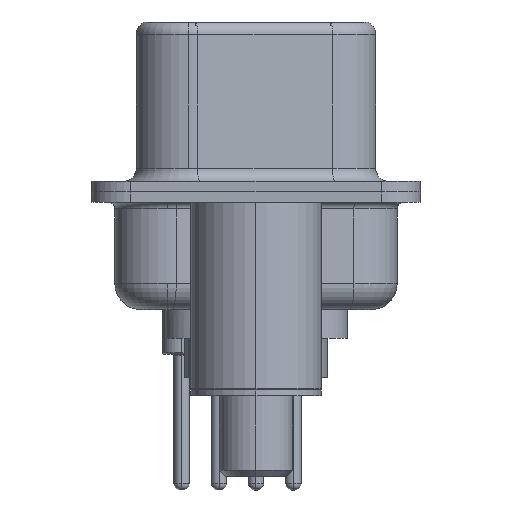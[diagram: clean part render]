
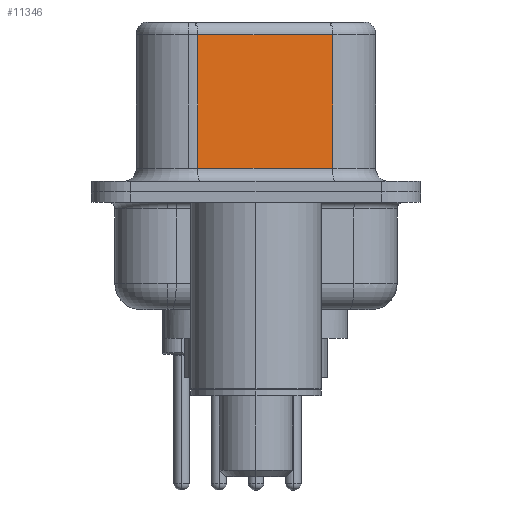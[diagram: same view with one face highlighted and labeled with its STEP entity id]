
A CAD part, left-side view. The second image highlights one B-rep face of the part: STEP entity #11346.
In plain terms, the highlighted planar face has unit normal (-0.985, -0.174, 0).
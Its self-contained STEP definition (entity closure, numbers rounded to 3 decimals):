
#1981 = FACE_OUTER_BOUND ( 'NONE', #14353, .T. ) ;
#3044 = LINE ( 'NONE', #11642, #13632 ) ;
#3157 = CARTESIAN_POINT ( 'NONE',  ( 4.58, -2.927, 0.9 ) ) ;
#3682 = EDGE_CURVE ( 'NONE', #15839, #12883, #19473, .T. ) ;
#4024 = DIRECTION ( 'NONE',  ( 0.985, 0.174, 0. ) ) ;
#4207 = CARTESIAN_POINT ( 'NONE',  ( 3.67, 2.233, 6.52 ) ) ;
#5188 = VECTOR ( 'NONE', #8578, 1000. ) ;
#5780 = LINE ( 'NONE', #6687, #5188 ) ;
#6687 = CARTESIAN_POINT ( 'NONE',  ( 4.58, -2.927, 6.02 ) ) ;
#6841 = ORIENTED_EDGE ( 'NONE', *, *, #12489, .T. ) ;
#6988 = VERTEX_POINT ( 'NONE', #14162 ) ;
#8578 = DIRECTION ( 'NONE',  ( -0.174, 0.985, 0. ) ) ;
#9517 = CARTESIAN_POINT ( 'NONE',  ( 4.58, -2.927, 6.52 ) ) ;
#10070 = CARTESIAN_POINT ( 'NONE',  ( 4.58, -2.927, 6.02 ) ) ;
#11021 = VECTOR ( 'NONE', #21347, 1000. ) ;
#11346 = ADVANCED_FACE ( 'NONE', ( #1981 ), #11503, .F. ) ;
#11503 = PLANE ( 'NONE',  #18878 ) ;
#11642 = CARTESIAN_POINT ( 'NONE',  ( 4.58, -2.927, 0.9 ) ) ;
#12027 = ORIENTED_EDGE ( 'NONE', *, *, #23517, .T. ) ;
#12489 = EDGE_CURVE ( 'NONE', #6988, #12883, #3044, .T. ) ;
#12883 = VERTEX_POINT ( 'NONE', #3157 ) ;
#13344 = DIRECTION ( 'NONE',  ( 0., 0., -1. ) ) ;
#13632 = VECTOR ( 'NONE', #23105, 1000. ) ;
#13852 = VECTOR ( 'NONE', #13344, 1000. ) ;
#14162 = CARTESIAN_POINT ( 'NONE',  ( 3.67, 2.233, 0.9 ) ) ;
#14353 = EDGE_LOOP ( 'NONE', ( #14445, #12027, #16036, #6841 ) ) ;
#14445 = ORIENTED_EDGE ( 'NONE', *, *, #3682, .F. ) ;
#15839 = VERTEX_POINT ( 'NONE', #10070 ) ;
#16036 = ORIENTED_EDGE ( 'NONE', *, *, #17148, .T. ) ;
#16048 = LINE ( 'NONE', #4207, #11021 ) ;
#17148 = EDGE_CURVE ( 'NONE', #23911, #6988, #16048, .T. ) ;
#17184 = DIRECTION ( 'NONE',  ( -0.174, 0.985, 0. ) ) ;
#17306 = CARTESIAN_POINT ( 'NONE',  ( 3.67, 2.233, 6.02 ) ) ;
#17899 = CARTESIAN_POINT ( 'NONE',  ( 4.58, -2.927, 6.52 ) ) ;
#18878 = AXIS2_PLACEMENT_3D ( 'NONE', #9517, #4024, #17184 ) ;
#19473 = LINE ( 'NONE', #17899, #13852 ) ;
#21347 = DIRECTION ( 'NONE',  ( 0., 0., -1. ) ) ;
#23105 = DIRECTION ( 'NONE',  ( 0.174, -0.985, 0. ) ) ;
#23517 = EDGE_CURVE ( 'NONE', #15839, #23911, #5780, .T. ) ;
#23911 = VERTEX_POINT ( 'NONE', #17306 ) ;
